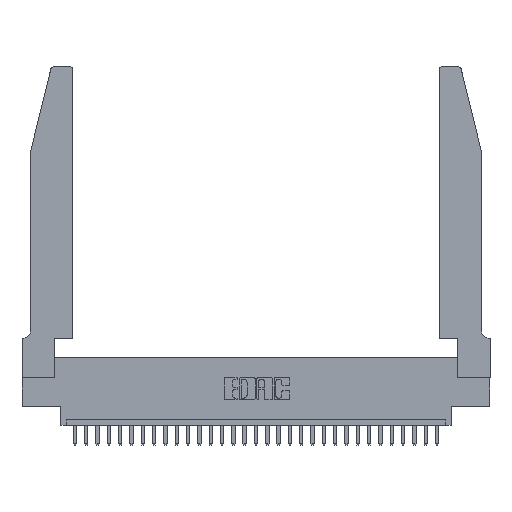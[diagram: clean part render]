
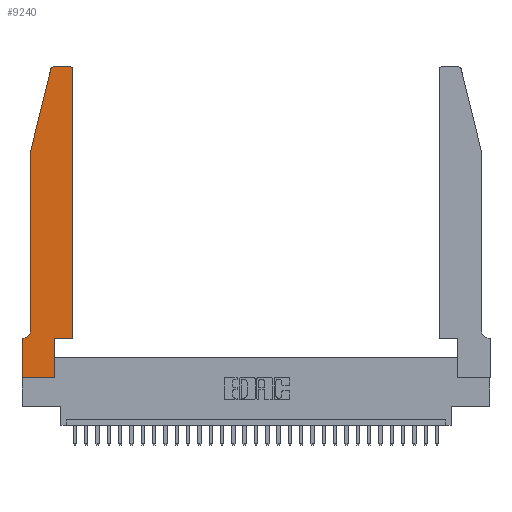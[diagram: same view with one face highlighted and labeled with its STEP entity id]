
A CAD part, top view. The second image highlights one B-rep face of the part: STEP entity #9240.
In plain terms, the highlighted planar face has unit normal (0, 0, 1).
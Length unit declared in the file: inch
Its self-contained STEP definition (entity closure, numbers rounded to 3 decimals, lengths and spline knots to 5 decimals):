
#404 = CARTESIAN_POINT ( 'NONE',  ( 0.2865, 0.35, 0.37 ) ) ;
#1361 = VERTEX_POINT ( 'NONE', #20550 ) ;
#1511 = VERTEX_POINT ( 'NONE', #8626 ) ;
#1779 = EDGE_CURVE ( 'NONE', #1361, #28480, #15244, .T. ) ;
#1786 = DIRECTION ( 'NONE',  ( 0., 0., 1. ) ) ;
#1832 = VERTEX_POINT ( 'NONE', #12730 ) ;
#2401 = VECTOR ( 'NONE', #27059, 39.37008 ) ;
#3034 = DIRECTION ( 'NONE',  ( 1., 0., 0. ) ) ;
#3147 = LINE ( 'NONE', #22065, #2401 ) ;
#3538 = CARTESIAN_POINT ( 'NONE',  ( 0.2605, 2.75, 0.37 ) ) ;
#4033 = CARTESIAN_POINT ( 'NONE',  ( 0.0055, 0.42, 0.37 ) ) ;
#4517 = VERTEX_POINT ( 'NONE', #27202 ) ;
#4638 = EDGE_CURVE ( 'NONE', #25368, #15389, #28072, .T. ) ;
#4995 = LINE ( 'NONE', #18207, #27127 ) ;
#5187 = DIRECTION ( 'NONE',  ( 0., 0., 1. ) ) ;
#5208 = EDGE_CURVE ( 'NONE', #15389, #21543, #11635, .T. ) ;
#5245 = CARTESIAN_POINT ( 'NONE',  ( 0.284, 2.75, 0.37 ) ) ;
#5346 = ORIENTED_EDGE ( 'NONE', *, *, #1779, .T. ) ;
#5526 = CARTESIAN_POINT ( 'NONE',  ( 0.4205, 2.72, 0.37 ) ) ;
#5723 = CARTESIAN_POINT ( 'NONE',  ( 0.4205, 2.75, 0.37 ) ) ;
#5906 = VERTEX_POINT ( 'NONE', #21352 ) ;
#6706 = EDGE_CURVE ( 'NONE', #9934, #1511, #18360, .T. ) ;
#7669 = FACE_OUTER_BOUND ( 'NONE', #25122, .T. ) ;
#7859 = DIRECTION ( 'NONE',  ( 1., 0., 0. ) ) ;
#8305 = DIRECTION ( 'NONE',  ( 0., -1., 0. ) ) ;
#8626 = CARTESIAN_POINT ( 'NONE',  ( 0.25487, 2.72718, 0.37 ) ) ;
#9240 = ADVANCED_FACE ( 'NONE', ( #7669 ), #26527, .T. ) ;
#9364 = EDGE_CURVE ( 'NONE', #4517, #1361, #4995, .T. ) ;
#9631 = ORIENTED_EDGE ( 'NONE', *, *, #20075, .T. ) ;
#9795 = CARTESIAN_POINT ( 'NONE',  ( 0., 0., 0.37 ) ) ;
#9934 = VERTEX_POINT ( 'NONE', #5245 ) ;
#10231 = DIRECTION ( 'NONE',  ( 0., 1., 0. ) ) ;
#10528 = VECTOR ( 'NONE', #17360, 39.37008 ) ;
#10551 = CARTESIAN_POINT ( 'NONE',  ( 0.0755, 2., 0.37 ) ) ;
#11054 = VECTOR ( 'NONE', #10231, 39.37008 ) ;
#11635 = LINE ( 'NONE', #9795, #13929 ) ;
#11759 = ORIENTED_EDGE ( 'NONE', *, *, #6706, .T. ) ;
#11861 = EDGE_CURVE ( 'NONE', #5906, #18960, #13968, .T. ) ;
#12730 = CARTESIAN_POINT ( 'NONE',  ( 0.2865, 0.35, 0.37 ) ) ;
#13118 = DIRECTION ( 'NONE',  ( 0., 1., 0. ) ) ;
#13929 = VECTOR ( 'NONE', #26574, 39.37008 ) ;
#13968 = CIRCLE ( 'NONE', #29675, 0.07 ) ;
#13974 = ORIENTED_EDGE ( 'NONE', *, *, #4638, .T. ) ;
#14368 = VECTOR ( 'NONE', #26943, 39.37008 ) ;
#14482 = CARTESIAN_POINT ( 'NONE',  ( 0., 0.35, 0.37 ) ) ;
#14797 = EDGE_CURVE ( 'NONE', #28480, #9934, #20039, .T. ) ;
#14867 = VECTOR ( 'NONE', #3034, 39.37008 ) ;
#15094 = CARTESIAN_POINT ( 'NONE',  ( 0.284, 2.72, 0.37 ) ) ;
#15244 = CIRCLE ( 'NONE', #29314, 0.03 ) ;
#15329 = CARTESIAN_POINT ( 'NONE',  ( 0.0055, 0.35, 0.37 ) ) ;
#15389 = VERTEX_POINT ( 'NONE', #28619 ) ;
#15651 = DIRECTION ( 'NONE',  ( -1., 0., 0. ) ) ;
#16026 = VECTOR ( 'NONE', #8305, 39.37008 ) ;
#16098 = DIRECTION ( 'NONE',  ( 1., 0., 0. ) ) ;
#16542 = VERTEX_POINT ( 'NONE', #28021 ) ;
#16765 = ORIENTED_EDGE ( 'NONE', *, *, #11861, .T. ) ;
#16946 = DIRECTION ( 'NONE',  ( -1., 0., 0. ) ) ;
#17360 = DIRECTION ( 'NONE',  ( 0., -1., 0. ) ) ;
#17842 = DIRECTION ( 'NONE',  ( 0., 0., 1. ) ) ;
#18207 = CARTESIAN_POINT ( 'NONE',  ( 0.4505, 0.35, 0.37 ) ) ;
#18208 = EDGE_CURVE ( 'NONE', #1832, #4517, #20069, .T. ) ;
#18360 = CIRCLE ( 'NONE', #29980, 0.03 ) ;
#18960 = VERTEX_POINT ( 'NONE', #15329 ) ;
#19118 = EDGE_CURVE ( 'NONE', #1511, #16542, #3147, .T. ) ;
#19642 = VECTOR ( 'NONE', #15651, 39.37008 ) ;
#19680 = ORIENTED_EDGE ( 'NONE', *, *, #19118, .T. ) ;
#20020 = AXIS2_PLACEMENT_3D ( 'NONE', #14482, #5187, #24374 ) ;
#20039 = LINE ( 'NONE', #3538, #19642 ) ;
#20069 = LINE ( 'NONE', #29854, #14867 ) ;
#20075 = EDGE_CURVE ( 'NONE', #21543, #1832, #30850, .T. ) ;
#20550 = CARTESIAN_POINT ( 'NONE',  ( 0.4505, 2.72, 0.37 ) ) ;
#21119 = CARTESIAN_POINT ( 'NONE',  ( 0., 0.35, 0.37 ) ) ;
#21333 = ORIENTED_EDGE ( 'NONE', *, *, #28914, .T. ) ;
#21352 = CARTESIAN_POINT ( 'NONE',  ( 0.0755, 0.42, 0.37 ) ) ;
#21543 = VERTEX_POINT ( 'NONE', #28293 ) ;
#21619 = DIRECTION ( 'NONE',  ( 0., 0., -1. ) ) ;
#22065 = CARTESIAN_POINT ( 'NONE',  ( 0.0755, 2., 0.37 ) ) ;
#23705 = LINE ( 'NONE', #29486, #14368 ) ;
#23997 = ORIENTED_EDGE ( 'NONE', *, *, #26277, .T. ) ;
#24374 = DIRECTION ( 'NONE',  ( 1., 0., 0. ) ) ;
#24562 = ORIENTED_EDGE ( 'NONE', *, *, #9364, .T. ) ;
#25013 = ORIENTED_EDGE ( 'NONE', *, *, #18208, .T. ) ;
#25122 = EDGE_LOOP ( 'NONE', ( #29862, #11759, #19680, #23997, #16765, #21333, #13974, #28915, #9631, #25013, #24562, #5346 ) ) ;
#25368 = VERTEX_POINT ( 'NONE', #21119 ) ;
#26277 = EDGE_CURVE ( 'NONE', #16542, #5906, #30955, .T. ) ;
#26527 = PLANE ( 'NONE',  #20020 ) ;
#26574 = DIRECTION ( 'NONE',  ( 1., 0., 0. ) ) ;
#26943 = DIRECTION ( 'NONE',  ( -1., 0., 0. ) ) ;
#27059 = DIRECTION ( 'NONE',  ( -0.239, -0.971, 0. ) ) ;
#27127 = VECTOR ( 'NONE', #13118, 39.37008 ) ;
#27202 = CARTESIAN_POINT ( 'NONE',  ( 0.4505, 0.35, 0.37 ) ) ;
#28021 = CARTESIAN_POINT ( 'NONE',  ( 0.0755, 2., 0.37 ) ) ;
#28072 = LINE ( 'NONE', #29044, #10528 ) ;
#28293 = CARTESIAN_POINT ( 'NONE',  ( 0.2865, 0., 0.37 ) ) ;
#28480 = VERTEX_POINT ( 'NONE', #5723 ) ;
#28619 = CARTESIAN_POINT ( 'NONE',  ( 0., 0., 0.37 ) ) ;
#28914 = EDGE_CURVE ( 'NONE', #18960, #25368, #23705, .T. ) ;
#28915 = ORIENTED_EDGE ( 'NONE', *, *, #5208, .T. ) ;
#29044 = CARTESIAN_POINT ( 'NONE',  ( 0., 0., 0.37 ) ) ;
#29314 = AXIS2_PLACEMENT_3D ( 'NONE', #5526, #17842, #7859 ) ;
#29486 = CARTESIAN_POINT ( 'NONE',  ( 0.0755, 0.35, 0.37 ) ) ;
#29675 = AXIS2_PLACEMENT_3D ( 'NONE', #4033, #21619, #16946 ) ;
#29854 = CARTESIAN_POINT ( 'NONE',  ( 0.4505, 0.35, 0.37 ) ) ;
#29862 = ORIENTED_EDGE ( 'NONE', *, *, #14797, .T. ) ;
#29980 = AXIS2_PLACEMENT_3D ( 'NONE', #15094, #1786, #16098 ) ;
#30850 = LINE ( 'NONE', #404, #11054 ) ;
#30955 = LINE ( 'NONE', #10551, #16026 ) ;
